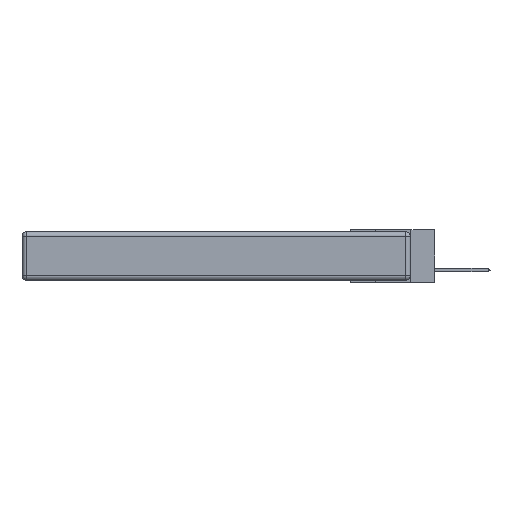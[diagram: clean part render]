
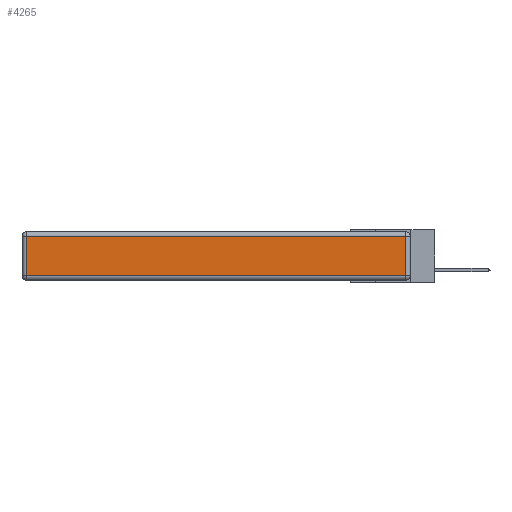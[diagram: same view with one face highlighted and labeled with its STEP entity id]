
A CAD part, left-side view. The second image highlights one B-rep face of the part: STEP entity #4265.
In plain terms, the highlighted planar face has unit normal (-1, 0, 0).
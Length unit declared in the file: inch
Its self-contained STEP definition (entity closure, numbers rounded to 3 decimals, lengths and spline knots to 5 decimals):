
#1065 = CARTESIAN_POINT ( 'NONE',  ( 0., 0., -0.313 ) ) ;
#1414 = ORIENTED_EDGE ( 'NONE', *, *, #1558, .T. ) ;
#1558 = EDGE_CURVE ( 'NONE', #4332, #18145, #15846, .T. ) ;
#2236 = EDGE_CURVE ( 'NONE', #2668, #4414, #13518, .T. ) ;
#2637 = EDGE_CURVE ( 'NONE', #18145, #2668, #11758, .T. ) ;
#2668 = VERTEX_POINT ( 'NONE', #22628 ) ;
#3064 = CARTESIAN_POINT ( 'NONE',  ( 0., 0.03, -0.343 ) ) ;
#4265 = ADVANCED_FACE ( 'NONE', ( #5891 ), #16567, .T. ) ;
#4332 = VERTEX_POINT ( 'NONE', #14651 ) ;
#4399 = AXIS2_PLACEMENT_3D ( 'NONE', #18410, #9210, #5693 ) ;
#4414 = VERTEX_POINT ( 'NONE', #6091 ) ;
#5693 = DIRECTION ( 'NONE',  ( 0., 0., 1. ) ) ;
#5891 = FACE_OUTER_BOUND ( 'NONE', #10987, .T. ) ;
#6091 = CARTESIAN_POINT ( 'NONE',  ( 0., 0.03, -0.313 ) ) ;
#6799 = DIRECTION ( 'NONE',  ( 0., -1., 0. ) ) ;
#7956 = CARTESIAN_POINT ( 'NONE',  ( 0., 2.72, -0.03 ) ) ;
#8646 = DIRECTION ( 'NONE',  ( 0., 0., 1. ) ) ;
#9210 = DIRECTION ( 'NONE',  ( -1., 0., 0. ) ) ;
#9564 = EDGE_CURVE ( 'NONE', #4414, #4332, #15548, .T. ) ;
#9663 = CARTESIAN_POINT ( 'NONE',  ( 0., 2.72, -0.343 ) ) ;
#10987 = EDGE_LOOP ( 'NONE', ( #22858, #15369, #1414, #23149 ) ) ;
#11009 = VECTOR ( 'NONE', #15080, 39.37008 ) ;
#11758 = LINE ( 'NONE', #9663, #15773 ) ;
#13131 = CARTESIAN_POINT ( 'NONE',  ( 0., 2.75, -0.03 ) ) ;
#13518 = LINE ( 'NONE', #1065, #14365 ) ;
#14365 = VECTOR ( 'NONE', #6799, 39.37008 ) ;
#14651 = CARTESIAN_POINT ( 'NONE',  ( 0., 0.03, -0.03 ) ) ;
#15080 = DIRECTION ( 'NONE',  ( 0., 1., 0. ) ) ;
#15369 = ORIENTED_EDGE ( 'NONE', *, *, #9564, .T. ) ;
#15548 = LINE ( 'NONE', #3064, #21300 ) ;
#15773 = VECTOR ( 'NONE', #17086, 39.37008 ) ;
#15846 = LINE ( 'NONE', #13131, #11009 ) ;
#16567 = PLANE ( 'NONE',  #4399 ) ;
#17086 = DIRECTION ( 'NONE',  ( 0., 0., -1. ) ) ;
#18145 = VERTEX_POINT ( 'NONE', #7956 ) ;
#18410 = CARTESIAN_POINT ( 'NONE',  ( 0., 0., -0.343 ) ) ;
#21300 = VECTOR ( 'NONE', #8646, 39.37008 ) ;
#22628 = CARTESIAN_POINT ( 'NONE',  ( 0., 2.72, -0.313 ) ) ;
#22858 = ORIENTED_EDGE ( 'NONE', *, *, #2236, .T. ) ;
#23149 = ORIENTED_EDGE ( 'NONE', *, *, #2637, .T. ) ;
